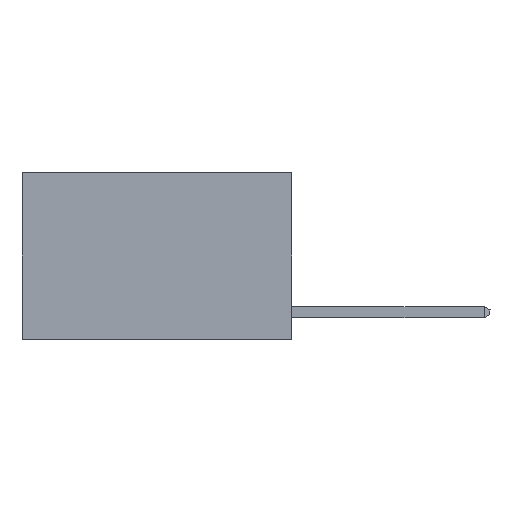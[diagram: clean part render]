
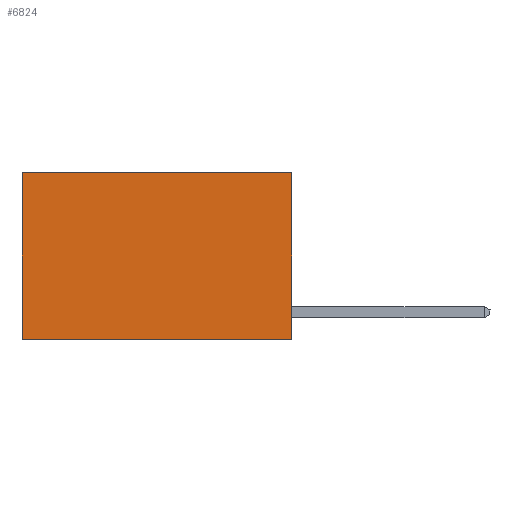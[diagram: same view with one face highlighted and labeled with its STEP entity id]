
A CAD part, left-side view. The second image highlights one B-rep face of the part: STEP entity #6824.
In plain terms, the highlighted planar face has unit normal (-1, 0, 0).
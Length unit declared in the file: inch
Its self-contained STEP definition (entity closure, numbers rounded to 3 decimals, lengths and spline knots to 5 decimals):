
#80 = CARTESIAN_POINT ( 'NONE',  ( 0.2625, 0., -0.37 ) ) ;
#1091 = CARTESIAN_POINT ( 'NONE',  ( 0.2625, 0.6, 0. ) ) ;
#1104 = EDGE_CURVE ( 'NONE', #4843, #1347, #6085, .T. ) ;
#1347 = VERTEX_POINT ( 'NONE', #11811 ) ;
#1991 = LINE ( 'NONE', #4242, #4300 ) ;
#2110 = LINE ( 'NONE', #1091, #7109 ) ;
#2279 = LINE ( 'NONE', #8857, #12375 ) ;
#2316 = PLANE ( 'NONE',  #9911 ) ;
#2530 = EDGE_CURVE ( 'NONE', #6524, #10726, #2279, .T. ) ;
#3100 = DIRECTION ( 'NONE',  ( 0., 0., -1. ) ) ;
#3300 = CARTESIAN_POINT ( 'NONE',  ( 0.2625, 0., 0. ) ) ;
#3862 = CARTESIAN_POINT ( 'NONE',  ( 0.2625, 0., 0. ) ) ;
#4149 = EDGE_CURVE ( 'NONE', #1347, #10726, #2110, .T. ) ;
#4242 = CARTESIAN_POINT ( 'NONE',  ( 0.2625, 0., 0. ) ) ;
#4280 = DIRECTION ( 'NONE',  ( 0., 0., -1. ) ) ;
#4300 = VECTOR ( 'NONE', #5251, 39.37008 ) ;
#4843 = VERTEX_POINT ( 'NONE', #3862 ) ;
#4995 = FACE_OUTER_BOUND ( 'NONE', #9845, .T. ) ;
#5083 = ORIENTED_EDGE ( 'NONE', *, *, #4149, .T. ) ;
#5251 = DIRECTION ( 'NONE',  ( 0., 0., -1. ) ) ;
#5433 = VECTOR ( 'NONE', #6563, 39.37008 ) ;
#5665 = ORIENTED_EDGE ( 'NONE', *, *, #9273, .F. ) ;
#5863 = ORIENTED_EDGE ( 'NONE', *, *, #2530, .F. ) ;
#6085 = LINE ( 'NONE', #8095, #5433 ) ;
#6524 = VERTEX_POINT ( 'NONE', #80 ) ;
#6563 = DIRECTION ( 'NONE',  ( 0., 1., 0. ) ) ;
#6740 = ORIENTED_EDGE ( 'NONE', *, *, #1104, .T. ) ;
#6824 = ADVANCED_FACE ( 'NONE', ( #4995 ), #2316, .F. ) ;
#7064 = DIRECTION ( 'NONE',  ( 0., 1., 0. ) ) ;
#7109 = VECTOR ( 'NONE', #3100, 39.37008 ) ;
#8095 = CARTESIAN_POINT ( 'NONE',  ( 0.2625, 0., 0. ) ) ;
#8857 = CARTESIAN_POINT ( 'NONE',  ( 0.2625, 0., -0.37 ) ) ;
#9273 = EDGE_CURVE ( 'NONE', #4843, #6524, #1991, .T. ) ;
#9845 = EDGE_LOOP ( 'NONE', ( #5083, #5863, #5665, #6740 ) ) ;
#9911 = AXIS2_PLACEMENT_3D ( 'NONE', #3300, #10304, #4280 ) ;
#10304 = DIRECTION ( 'NONE',  ( 1., 0., 0. ) ) ;
#10726 = VERTEX_POINT ( 'NONE', #11051 ) ;
#11051 = CARTESIAN_POINT ( 'NONE',  ( 0.2625, 0.6, -0.37 ) ) ;
#11811 = CARTESIAN_POINT ( 'NONE',  ( 0.2625, 0.6, 0. ) ) ;
#12375 = VECTOR ( 'NONE', #7064, 39.37008 ) ;
